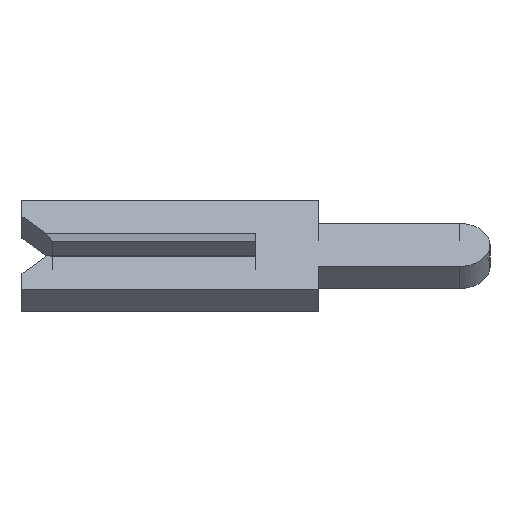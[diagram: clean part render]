
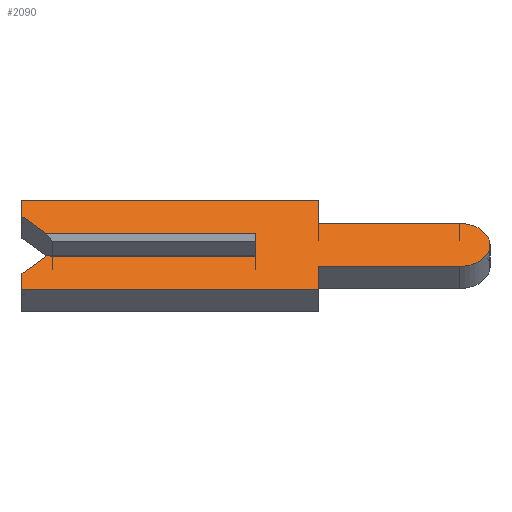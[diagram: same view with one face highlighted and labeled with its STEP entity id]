
A CAD part, left-side view. The second image highlights one B-rep face of the part: STEP entity #2090.
In plain terms, the highlighted face is planar.
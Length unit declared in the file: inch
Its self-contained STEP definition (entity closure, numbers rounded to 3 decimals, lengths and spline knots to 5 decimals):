
#4 = VECTOR ( 'NONE', #1769, 39.37008 ) ;
#22 = CARTESIAN_POINT ( 'NONE',  ( -0.01, -0.1305, -0.0195 ) ) ;
#34 = EDGE_CURVE ( 'NONE', #2298, #763, #2204, .T. ) ;
#78 = DIRECTION ( 'NONE',  ( 0., -1., 0. ) ) ;
#138 = ORIENTED_EDGE ( 'NONE', *, *, #1469, .F. ) ;
#146 = CARTESIAN_POINT ( 'NONE',  ( -0.01, -0.04, -0.0195 ) ) ;
#165 = EDGE_LOOP ( 'NONE', ( #2487, #1703, #1768, #1510, #1055, #861, #786, #138, #850, #1487, #1029, #2407, #2219, #2503 ) ) ;
#230 = LINE ( 'NONE', #1295, #1240 ) ;
#277 = VERTEX_POINT ( 'NONE', #1383 ) ;
#289 = CARTESIAN_POINT ( 'NONE',  ( -0.01, -0.1305, 0.0195 ) ) ;
#340 = EDGE_CURVE ( 'NONE', #423, #2041, #869, .T. ) ;
#374 = CARTESIAN_POINT ( 'NONE',  ( -0.01, -0.04, 0.0195 ) ) ;
#420 = CARTESIAN_POINT ( 'NONE',  ( -0.01, -0.04, 0.04 ) ) ;
#423 = VERTEX_POINT ( 'NONE', #1004 ) ;
#468 = LINE ( 'NONE', #880, #1922 ) ;
#484 = CARTESIAN_POINT ( 'NONE',  ( -0.01, -0.04, 0.0195 ) ) ;
#495 = LINE ( 'NONE', #146, #1913 ) ;
#531 = LINE ( 'NONE', #1899, #2208 ) ;
#553 = LINE ( 'NONE', #967, #1686 ) ;
#554 = DIRECTION ( 'NONE',  ( 0., 0., 1. ) ) ;
#566 = CARTESIAN_POINT ( 'NONE',  ( -0.01, 0.15, -0.026 ) ) ;
#571 = DIRECTION ( 'NONE',  ( 0., 0., -1. ) ) ;
#579 = CARTESIAN_POINT ( 'NONE',  ( -0.01, 0.15, -0.04 ) ) ;
#734 = EDGE_CURVE ( 'NONE', #2123, #2298, #1528, .T. ) ;
#759 = DIRECTION ( 'NONE',  ( 0., 0., -1. ) ) ;
#763 = VERTEX_POINT ( 'NONE', #22 ) ;
#786 = ORIENTED_EDGE ( 'NONE', *, *, #1394, .F. ) ;
#799 = DIRECTION ( 'NONE',  ( 0., 0., 1. ) ) ;
#850 = ORIENTED_EDGE ( 'NONE', *, *, #34, .F. ) ;
#861 = ORIENTED_EDGE ( 'NONE', *, *, #1387, .F. ) ;
#869 = LINE ( 'NONE', #1405, #1946 ) ;
#880 = CARTESIAN_POINT ( 'NONE',  ( -0.01, -0.1305, -0.01 ) ) ;
#890 = CARTESIAN_POINT ( 'NONE',  ( -0.01, 0.134, 0.01 ) ) ;
#894 = VECTOR ( 'NONE', #2588, 39.37008 ) ;
#912 = VERTEX_POINT ( 'NONE', #420 ) ;
#927 = VECTOR ( 'NONE', #2189, 39.37008 ) ;
#954 = LINE ( 'NONE', #1572, #2233 ) ;
#967 = CARTESIAN_POINT ( 'NONE',  ( -0.01, -0.04, -0.04 ) ) ;
#976 = DIRECTION ( 'NONE',  ( 0., 1., 0. ) ) ;
#990 = CARTESIAN_POINT ( 'NONE',  ( -0.01, -0.04, 0.04 ) ) ;
#1004 = CARTESIAN_POINT ( 'NONE',  ( -0.01, 0., -0.01 ) ) ;
#1029 = ORIENTED_EDGE ( 'NONE', *, *, #1245, .F. ) ;
#1055 = ORIENTED_EDGE ( 'NONE', *, *, #2422, .F. ) ;
#1132 = VERTEX_POINT ( 'NONE', #1842 ) ;
#1134 = CARTESIAN_POINT ( 'NONE',  ( -0.01, -0.04, -0.0195 ) ) ;
#1186 = CARTESIAN_POINT ( 'NONE',  ( -0.01, 0.15, 0.026 ) ) ;
#1240 = VECTOR ( 'NONE', #1281, 39.37008 ) ;
#1245 = EDGE_CURVE ( 'NONE', #912, #2123, #2106, .T. ) ;
#1270 = VERTEX_POINT ( 'NONE', #1389 ) ;
#1277 = EDGE_CURVE ( 'NONE', #1574, #277, #1471, .T. ) ;
#1281 = DIRECTION ( 'NONE',  ( 0., -1., 0. ) ) ;
#1295 = CARTESIAN_POINT ( 'NONE',  ( -0.01, 0.15, 0.04 ) ) ;
#1300 = DIRECTION ( 'NONE',  ( 0., -1., 0. ) ) ;
#1304 = FACE_OUTER_BOUND ( 'NONE', #165, .T. ) ;
#1312 = EDGE_CURVE ( 'NONE', #2280, #1574, #1970, .T. ) ;
#1315 = LINE ( 'NONE', #566, #2555 ) ;
#1321 = PLANE ( 'NONE',  #1892 ) ;
#1326 = EDGE_CURVE ( 'NONE', #2280, #2041, #954, .T. ) ;
#1383 = CARTESIAN_POINT ( 'NONE',  ( -0.01, 0.15, 0.04 ) ) ;
#1387 = EDGE_CURVE ( 'NONE', #1132, #1270, #2550, .T. ) ;
#1389 = CARTESIAN_POINT ( 'NONE',  ( -0.01, 0.15, -0.04 ) ) ;
#1394 = EDGE_CURVE ( 'NONE', #2334, #1132, #553, .T. ) ;
#1398 = CARTESIAN_POINT ( 'NONE',  ( -0.01, 0.134, -0.01 ) ) ;
#1405 = CARTESIAN_POINT ( 'NONE',  ( -0.01, 0., 0.0065 ) ) ;
#1455 = VERTEX_POINT ( 'NONE', #1398 ) ;
#1469 = EDGE_CURVE ( 'NONE', #763, #2334, #495, .T. ) ;
#1471 = LINE ( 'NONE', #1186, #2519 ) ;
#1487 = ORIENTED_EDGE ( 'NONE', *, *, #734, .F. ) ;
#1507 = DIRECTION ( 'NONE',  ( 1., 0., 0. ) ) ;
#1510 = ORIENTED_EDGE ( 'NONE', *, *, #2150, .F. ) ;
#1528 = LINE ( 'NONE', #374, #1750 ) ;
#1555 = DIRECTION ( 'NONE',  ( 1., 0., 0. ) ) ;
#1561 = CARTESIAN_POINT ( 'NONE',  ( -0.01, 0.15, 0.026 ) ) ;
#1566 = CARTESIAN_POINT ( 'NONE',  ( -0.01, -0.1305, 0. ) ) ;
#1572 = CARTESIAN_POINT ( 'NONE',  ( -0.01, 0.15, 0.01 ) ) ;
#1574 = VERTEX_POINT ( 'NONE', #1561 ) ;
#1686 = VECTOR ( 'NONE', #571, 39.37008 ) ;
#1688 = CARTESIAN_POINT ( 'NONE',  ( -0.01, 0., 0.01 ) ) ;
#1703 = ORIENTED_EDGE ( 'NONE', *, *, #340, .F. ) ;
#1738 = CARTESIAN_POINT ( 'NONE',  ( -0.01, 0.1305, 0.0065 ) ) ;
#1750 = VECTOR ( 'NONE', #1300, 39.37008 ) ;
#1768 = ORIENTED_EDGE ( 'NONE', *, *, #2199, .F. ) ;
#1769 = DIRECTION ( 'NONE',  ( 0., 1., 0. ) ) ;
#1842 = CARTESIAN_POINT ( 'NONE',  ( -0.01, -0.04, -0.04 ) ) ;
#1892 = AXIS2_PLACEMENT_3D ( 'NONE', #2341, #1507, #2103 ) ;
#1899 = CARTESIAN_POINT ( 'NONE',  ( -0.01, 0.1305, -0.0065 ) ) ;
#1913 = VECTOR ( 'NONE', #976, 39.37008 ) ;
#1922 = VECTOR ( 'NONE', #78, 39.37008 ) ;
#1946 = VECTOR ( 'NONE', #799, 39.37008 ) ;
#1955 = VERTEX_POINT ( 'NONE', #2433 ) ;
#1970 = LINE ( 'NONE', #1738, #894 ) ;
#1989 = DIRECTION ( 'NONE',  ( 0., -1., 0. ) ) ;
#2041 = VERTEX_POINT ( 'NONE', #1688 ) ;
#2082 = EDGE_CURVE ( 'NONE', #277, #912, #230, .T. ) ;
#2090 = ADVANCED_FACE ( 'NONE', ( #1304 ), #1321, .F. ) ;
#2103 = DIRECTION ( 'NONE',  ( 0., 0., -1. ) ) ;
#2106 = LINE ( 'NONE', #990, #927 ) ;
#2123 = VERTEX_POINT ( 'NONE', #484 ) ;
#2150 = EDGE_CURVE ( 'NONE', #1955, #1455, #531, .T. ) ;
#2182 = DIRECTION ( 'NONE',  ( 0., 0., 1. ) ) ;
#2189 = DIRECTION ( 'NONE',  ( 0., 0., -1. ) ) ;
#2199 = EDGE_CURVE ( 'NONE', #1455, #423, #468, .T. ) ;
#2204 = CIRCLE ( 'NONE', #2437, 0.0195 ) ;
#2208 = VECTOR ( 'NONE', #2533, 39.37008 ) ;
#2219 = ORIENTED_EDGE ( 'NONE', *, *, #1277, .F. ) ;
#2233 = VECTOR ( 'NONE', #1989, 39.37008 ) ;
#2280 = VERTEX_POINT ( 'NONE', #890 ) ;
#2298 = VERTEX_POINT ( 'NONE', #289 ) ;
#2334 = VERTEX_POINT ( 'NONE', #1134 ) ;
#2341 = CARTESIAN_POINT ( 'NONE',  ( -0.01, -0.1305, 0. ) ) ;
#2407 = ORIENTED_EDGE ( 'NONE', *, *, #2082, .F. ) ;
#2422 = EDGE_CURVE ( 'NONE', #1270, #1955, #1315, .T. ) ;
#2433 = CARTESIAN_POINT ( 'NONE',  ( -0.01, 0.15, -0.026 ) ) ;
#2437 = AXIS2_PLACEMENT_3D ( 'NONE', #1566, #1555, #759 ) ;
#2487 = ORIENTED_EDGE ( 'NONE', *, *, #1326, .T. ) ;
#2503 = ORIENTED_EDGE ( 'NONE', *, *, #1312, .F. ) ;
#2519 = VECTOR ( 'NONE', #2182, 39.37008 ) ;
#2533 = DIRECTION ( 'NONE',  ( 0., -0.707, 0.707 ) ) ;
#2550 = LINE ( 'NONE', #579, #4 ) ;
#2555 = VECTOR ( 'NONE', #554, 39.37008 ) ;
#2588 = DIRECTION ( 'NONE',  ( 0., 0.707, 0.707 ) ) ;
